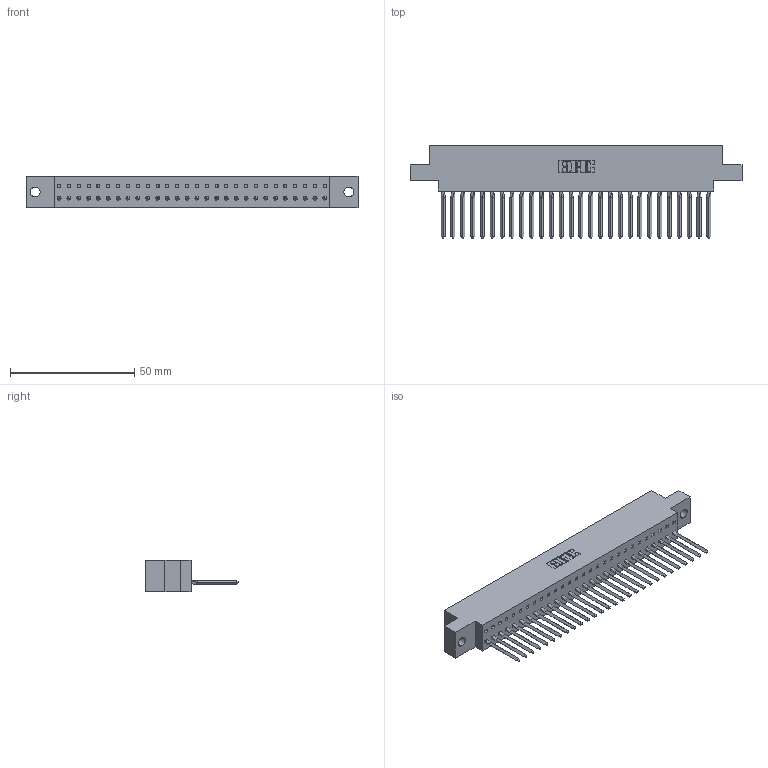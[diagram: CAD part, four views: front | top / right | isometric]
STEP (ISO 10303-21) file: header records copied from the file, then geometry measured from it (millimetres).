
FILE_DESCRIPTION (( 'STEP AP203' ), '1' );
FILE_NAME ('317-028-541-604.STEP', '2020-02-27T19:28:11', ( '' ), ( '' ), 'SwSTEP 2.0', 'SolidWorks 2016', '' );
FILE_SCHEMA (( 'CONFIG_CONTROL_DESIGN' ));
Length unit declared in the file: inch
Products named in the file (3): 317-028-541-604; 317 Part_.156 Dia - TH; 317-290-002_541
Assembly tree (29 placements, depth 2):
  317-028-541-604
    317 Part_.156 Dia - TH
    317-290-002_541  x28
Bounding box: 133.65 x 37.34 x 12.7 mm (x, y, z)
Volume: 21156 mm3; surface area: 29246.1 mm2
Topology: 29 solids, 29 shells, 4358 faces, 12427 edges, 8078 vertices
Faces by surface type: plane 3530, cylinder 716, bspline 112
Entity records: 43082 total; most frequent: CARTESIAN_POINT 8293, ORIENTED_EDGE 7574, DIRECTION 6211, EDGE_CURVE 3787, VECTOR 3423, LINE 3423, VERTEX_POINT 2516, AXIS2_PLACEMENT_3D 1394
